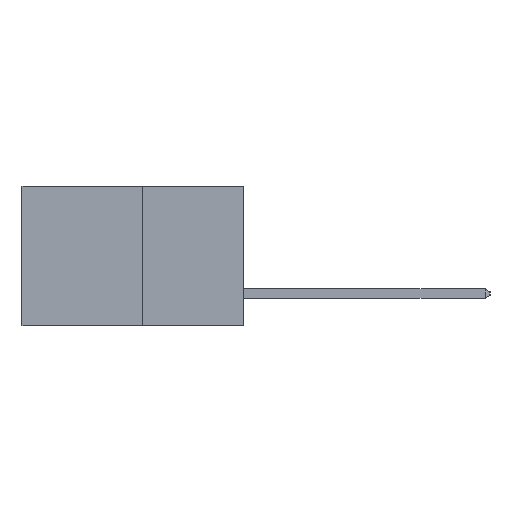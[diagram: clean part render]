
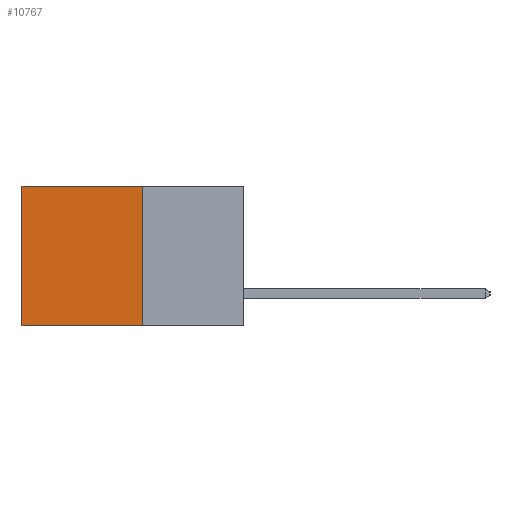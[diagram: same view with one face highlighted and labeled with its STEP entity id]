
A CAD part, left-side view. The second image highlights one B-rep face of the part: STEP entity #10767.
In plain terms, the highlighted planar face has unit normal (-1, 0, 0).
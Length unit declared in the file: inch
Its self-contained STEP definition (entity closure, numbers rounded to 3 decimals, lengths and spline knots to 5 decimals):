
#39 = EDGE_CURVE ( 'NONE', #9568, #3502, #6909, .T. ) ;
#401 = FACE_OUTER_BOUND ( 'NONE', #6630, .T. ) ;
#1105 = LINE ( 'NONE', #11065, #9999 ) ;
#1326 = AXIS2_PLACEMENT_3D ( 'NONE', #6815, #1540, #7694 ) ;
#1540 = DIRECTION ( 'NONE',  ( 1., 0., 0. ) ) ;
#1595 = CARTESIAN_POINT ( 'NONE',  ( 0.277, 0.59, -0.37 ) ) ;
#1979 = CARTESIAN_POINT ( 'NONE',  ( 0.277, 0.27, 0. ) ) ;
#1999 = VECTOR ( 'NONE', #3117, 39.37008 ) ;
#3117 = DIRECTION ( 'NONE',  ( 0., 1., 0. ) ) ;
#3451 = ORIENTED_EDGE ( 'NONE', *, *, #3905, .F. ) ;
#3502 = VERTEX_POINT ( 'NONE', #7458 ) ;
#3764 = DIRECTION ( 'NONE',  ( 0., 1., 0. ) ) ;
#3905 = EDGE_CURVE ( 'NONE', #8667, #9568, #1105, .T. ) ;
#3929 = CARTESIAN_POINT ( 'NONE',  ( 0.277, 0.27, -0.37 ) ) ;
#5232 = ORIENTED_EDGE ( 'NONE', *, *, #39, .F. ) ;
#6037 = ORIENTED_EDGE ( 'NONE', *, *, #8393, .T. ) ;
#6085 = LINE ( 'NONE', #1595, #6360 ) ;
#6360 = VECTOR ( 'NONE', #7749, 39.37008 ) ;
#6630 = EDGE_LOOP ( 'NONE', ( #7293, #5232, #3451, #6037 ) ) ;
#6732 = PLANE ( 'NONE',  #1326 ) ;
#6815 = CARTESIAN_POINT ( 'NONE',  ( 0.277, 0.27, -0.37 ) ) ;
#6909 = LINE ( 'NONE', #3929, #11031 ) ;
#7293 = ORIENTED_EDGE ( 'NONE', *, *, #8445, .T. ) ;
#7458 = CARTESIAN_POINT ( 'NONE',  ( 0.277, 0.59, -0.37 ) ) ;
#7491 = CARTESIAN_POINT ( 'NONE',  ( 0.277, 0.27, 0. ) ) ;
#7694 = DIRECTION ( 'NONE',  ( 0., 0., -1. ) ) ;
#7749 = DIRECTION ( 'NONE',  ( 0., 0., -1. ) ) ;
#8044 = CARTESIAN_POINT ( 'NONE',  ( 0.277, 0.59, 0. ) ) ;
#8393 = EDGE_CURVE ( 'NONE', #8667, #9291, #8885, .T. ) ;
#8445 = EDGE_CURVE ( 'NONE', #9291, #3502, #6085, .T. ) ;
#8468 = DIRECTION ( 'NONE',  ( 0., 0., -1. ) ) ;
#8667 = VERTEX_POINT ( 'NONE', #1979 ) ;
#8885 = LINE ( 'NONE', #7491, #1999 ) ;
#9291 = VERTEX_POINT ( 'NONE', #8044 ) ;
#9568 = VERTEX_POINT ( 'NONE', #10893 ) ;
#9999 = VECTOR ( 'NONE', #8468, 39.37008 ) ;
#10767 = ADVANCED_FACE ( 'NONE', ( #401 ), #6732, .F. ) ;
#10893 = CARTESIAN_POINT ( 'NONE',  ( 0.277, 0.27, -0.37 ) ) ;
#11031 = VECTOR ( 'NONE', #3764, 39.37008 ) ;
#11065 = CARTESIAN_POINT ( 'NONE',  ( 0.277, 0.27, -0.37 ) ) ;
